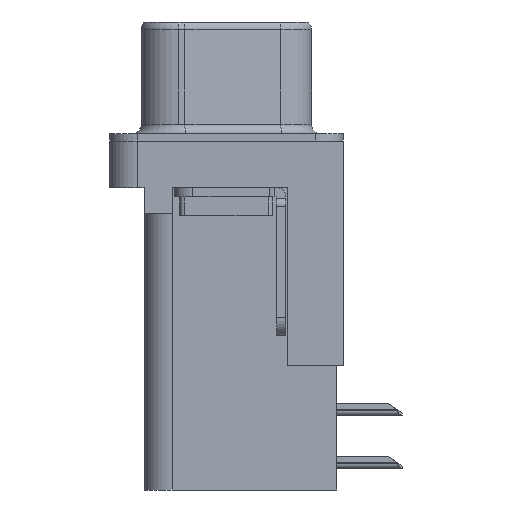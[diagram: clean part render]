
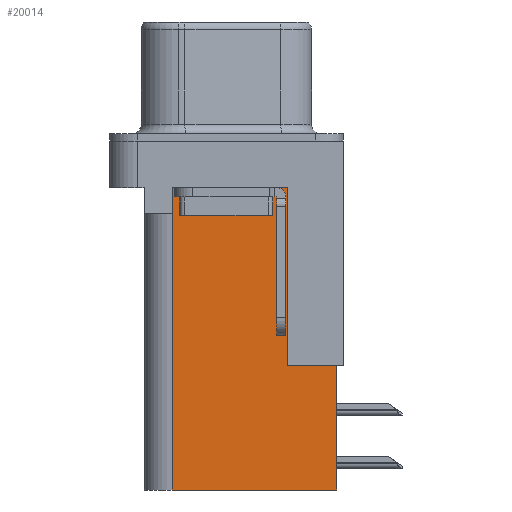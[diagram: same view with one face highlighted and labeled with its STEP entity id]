
A CAD part, left-side view. The second image highlights one B-rep face of the part: STEP entity #20014.
In plain terms, the highlighted planar face has unit normal (-1, 0, 0).
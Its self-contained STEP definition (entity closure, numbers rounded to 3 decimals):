
#560 = ORIENTED_EDGE ( 'NONE', *, *, #21375, .F. ) ;
#835 = VERTEX_POINT ( 'NONE', #22623 ) ;
#1445 = VECTOR ( 'NONE', #10568, 1000. ) ;
#2161 = VERTEX_POINT ( 'NONE', #16746 ) ;
#2293 = VECTOR ( 'NONE', #23015, 1000. ) ;
#2521 = VERTEX_POINT ( 'NONE', #17509 ) ;
#2549 = LINE ( 'NONE', #21182, #2293 ) ;
#2648 = VERTEX_POINT ( 'NONE', #3061 ) ;
#3061 = CARTESIAN_POINT ( 'NONE',  ( 3.79, 2.925, -3.9 ) ) ;
#4588 = CARTESIAN_POINT ( 'NONE',  ( 3.79, -3.295, -18.76 ) ) ;
#4828 = ORIENTED_EDGE ( 'NONE', *, *, #11448, .T. ) ;
#5359 = DIRECTION ( 'NONE',  ( 0., 0., 1. ) ) ;
#6069 = VECTOR ( 'NONE', #22920, 1000. ) ;
#6091 = LINE ( 'NONE', #15324, #6069 ) ;
#6109 = VERTEX_POINT ( 'NONE', #11143 ) ;
#6290 = ORIENTED_EDGE ( 'NONE', *, *, #21444, .T. ) ;
#6301 = FACE_OUTER_BOUND ( 'NONE', #22445, .T. ) ;
#6598 = DIRECTION ( 'NONE',  ( 1., 0., 0. ) ) ;
#6608 = VERTEX_POINT ( 'NONE', #11307 ) ;
#7246 = CARTESIAN_POINT ( 'NONE',  ( 3.79, -3.295, -2.5 ) ) ;
#8449 = PLANE ( 'NONE',  #20355 ) ;
#8554 = CARTESIAN_POINT ( 'NONE',  ( 3.79, 2.895, -3.9 ) ) ;
#8650 = CARTESIAN_POINT ( 'NONE',  ( 3.79, -5.925, -2. ) ) ;
#10024 = ORIENTED_EDGE ( 'NONE', *, *, #12456, .T. ) ;
#10553 = LINE ( 'NONE', #8554, #10621 ) ;
#10568 = DIRECTION ( 'NONE',  ( 0., 1., 0. ) ) ;
#10581 = EDGE_CURVE ( 'NONE', #13230, #6109, #15601, .T. ) ;
#10621 = VECTOR ( 'NONE', #16160, 1000. ) ;
#11001 = DIRECTION ( 'NONE',  ( 0., 1., 0. ) ) ;
#11143 = CARTESIAN_POINT ( 'NONE',  ( 3.79, 2.895, -2.5 ) ) ;
#11307 = CARTESIAN_POINT ( 'NONE',  ( 3.79, 2.925, -18.76 ) ) ;
#11448 = EDGE_CURVE ( 'NONE', #6109, #2521, #10553, .T. ) ;
#11557 = ORIENTED_EDGE ( 'NONE', *, *, #10581, .T. ) ;
#12456 = EDGE_CURVE ( 'NONE', #2521, #2648, #6091, .T. ) ;
#13230 = VERTEX_POINT ( 'NONE', #23914 ) ;
#13564 = ORIENTED_EDGE ( 'NONE', *, *, #22322, .T. ) ;
#13735 = ORIENTED_EDGE ( 'NONE', *, *, #21336, .F. ) ;
#13854 = VECTOR ( 'NONE', #5359, 1000. ) ;
#13907 = LINE ( 'NONE', #24100, #13854 ) ;
#13939 = VERTEX_POINT ( 'NONE', #18626 ) ;
#14110 = CARTESIAN_POINT ( 'NONE',  ( 3.79, -3.295, -18.76 ) ) ;
#14111 = ORIENTED_EDGE ( 'NONE', *, *, #20506, .F. ) ;
#15324 = CARTESIAN_POINT ( 'NONE',  ( 3.79, 0., -3.9 ) ) ;
#15574 = VECTOR ( 'NONE', #11001, 1000. ) ;
#15601 = LINE ( 'NONE', #7246, #15574 ) ;
#16160 = DIRECTION ( 'NONE',  ( 0., 0., -1. ) ) ;
#16746 = CARTESIAN_POINT ( 'NONE',  ( 3.79, -5.925, -12.05 ) ) ;
#17509 = CARTESIAN_POINT ( 'NONE',  ( 3.79, 2.895, -3.9 ) ) ;
#18270 = CARTESIAN_POINT ( 'NONE',  ( 3.79, -6.295, -12.05 ) ) ;
#18626 = CARTESIAN_POINT ( 'NONE',  ( 3.79, -5.925, -18.76 ) ) ;
#19913 = DIRECTION ( 'NONE',  ( 0., 1., 0. ) ) ;
#20014 = ADVANCED_FACE ( 'NONE', ( #6301 ), #8449, .F. ) ;
#20355 = AXIS2_PLACEMENT_3D ( 'NONE', #14110, #6598, #19913 ) ;
#20506 = EDGE_CURVE ( 'NONE', #6608, #2648, #2549, .T. ) ;
#20838 = VECTOR ( 'NONE', #21862, 1000. ) ;
#20860 = LINE ( 'NONE', #18270, #1445 ) ;
#20883 = LINE ( 'NONE', #8650, #20838 ) ;
#21074 = VECTOR ( 'NONE', #23529, 1000. ) ;
#21147 = LINE ( 'NONE', #4588, #21074 ) ;
#21182 = CARTESIAN_POINT ( 'NONE',  ( 3.79, 2.925, -18.76 ) ) ;
#21336 = EDGE_CURVE ( 'NONE', #13939, #6608, #21147, .T. ) ;
#21375 = EDGE_CURVE ( 'NONE', #2161, #13939, #20883, .T. ) ;
#21444 = EDGE_CURVE ( 'NONE', #2161, #835, #20860, .T. ) ;
#21862 = DIRECTION ( 'NONE',  ( 0., 0., -1. ) ) ;
#22322 = EDGE_CURVE ( 'NONE', #835, #13230, #13907, .T. ) ;
#22445 = EDGE_LOOP ( 'NONE', ( #11557, #4828, #10024, #14111, #13735, #560, #6290, #13564 ) ) ;
#22623 = CARTESIAN_POINT ( 'NONE',  ( 3.79, -3.295, -12.05 ) ) ;
#22920 = DIRECTION ( 'NONE',  ( 0., 1., 0. ) ) ;
#23015 = DIRECTION ( 'NONE',  ( 0., 0., 1. ) ) ;
#23529 = DIRECTION ( 'NONE',  ( 0., 1., 0. ) ) ;
#23914 = CARTESIAN_POINT ( 'NONE',  ( 3.79, -3.295, -2.5 ) ) ;
#24100 = CARTESIAN_POINT ( 'NONE',  ( 3.79, -3.295, -18.76 ) ) ;
